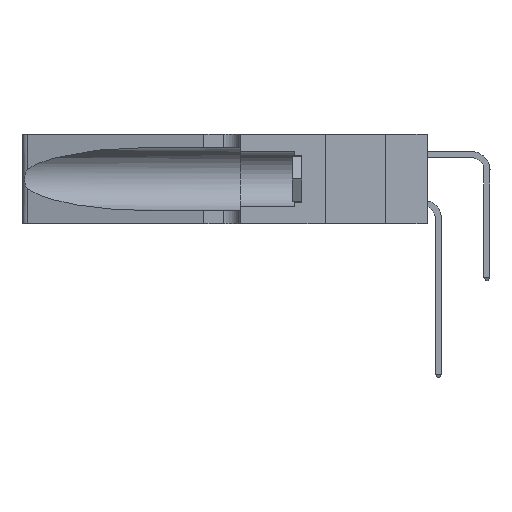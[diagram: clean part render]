
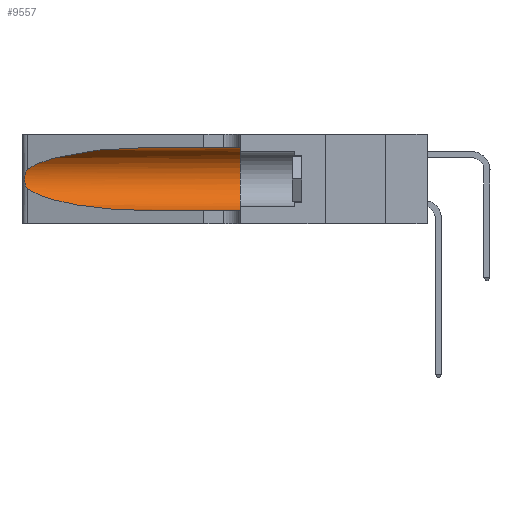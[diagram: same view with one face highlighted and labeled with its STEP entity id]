
A CAD part, left-side view. The second image highlights one B-rep face of the part: STEP entity #9557.
In plain terms, the highlighted cylindrical face has radius 3.308 mm (diameter 6.617 mm), a partial arc.
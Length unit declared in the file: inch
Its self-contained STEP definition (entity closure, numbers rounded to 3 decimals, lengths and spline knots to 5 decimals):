
#128 = DIRECTION ( 'NONE',  ( 0., -1., 0. ) ) ;
#168 = VERTEX_POINT ( 'NONE', #22204 ) ;
#1354 = CYLINDRICAL_SURFACE ( 'NONE', #5959, 0.13025 ) ;
#1761 = DIRECTION ( 'NONE',  ( 0., 1., 0. ) ) ;
#2140 = ORIENTED_EDGE ( 'NONE', *, *, #6679, .T. ) ;
#2148 = VERTEX_POINT ( 'NONE', #20950 ) ;
#2227 = CARTESIAN_POINT ( 'NONE',  ( 0.26018, 1.23835, 0.19895 ) ) ;
#3021 = VECTOR ( 'NONE', #128, 39.37008 ) ;
#3131 = DIRECTION ( 'NONE',  ( 0., 0., -1. ) ) ;
#3264 = VERTEX_POINT ( 'NONE', #19180 ) ;
#4527 = CARTESIAN_POINT ( 'NONE',  ( 0.25487, 1.22718, 0.22369 ) ) ;
#4631 = FACE_OUTER_BOUND ( 'NONE', #27424, .T. ) ;
#5343 =( BOUNDED_CURVE ( )  B_SPLINE_CURVE ( 3, ( #19104, #28848, #7785, #18140 ),
 .UNSPECIFIED., .F., .T. ) 
 B_SPLINE_CURVE_WITH_KNOTS ( ( 4, 4 ),
 ( 3.44316, 4.71239 ),
 .UNSPECIFIED. ) 
 CURVE ( )  GEOMETRIC_REPRESENTATION_ITEM ( )  RATIONAL_B_SPLINE_CURVE ( ( 1., 0.87, 0.87, 1. ) ) 
 REPRESENTATION_ITEM ( '' )  );
#5732 = CARTESIAN_POINT ( 'NONE',  ( 0.1305, 0.72297, 0.05475 ) ) ;
#5959 = AXIS2_PLACEMENT_3D ( 'NONE', #11702, #17139, #3131 ) ;
#6679 = EDGE_CURVE ( 'NONE', #9902, #25562, #5343, .T. ) ;
#6950 = CARTESIAN_POINT ( 'NONE',  ( 0.2373, 1.15595, 0.28018 ) ) ;
#7373 = CARTESIAN_POINT ( 'NONE',  ( 0.25856, 1.23593, 0.16098 ) ) ;
#7451 = CARTESIAN_POINT ( 'NONE',  ( 0.1305, 1.61858, 0.05475 ) ) ;
#7481 = ORIENTED_EDGE ( 'NONE', *, *, #14138, .T. ) ;
#7785 = CARTESIAN_POINT ( 'NONE',  ( 0.18966, 0.96281, 0.05475 ) ) ;
#9509 = CARTESIAN_POINT ( 'NONE',  ( 0.25639, 1.23184, 0.21858 ) ) ;
#9557 = ADVANCED_FACE ( 'NONE', ( #4631 ), #1354, .F. ) ;
#9620 = CARTESIAN_POINT ( 'NONE',  ( 0.25639, 1.23186, 0.15144 ) ) ;
#9720 = CARTESIAN_POINT ( 'NONE',  ( 0.25487, 1.22718, 0.22369 ) ) ;
#9807 = DIRECTION ( 'NONE',  ( 0., -1., 0. ) ) ;
#9902 = VERTEX_POINT ( 'NONE', #14813 ) ;
#10667 = ORIENTED_EDGE ( 'NONE', *, *, #11576, .T. ) ;
#10798 = CARTESIAN_POINT ( 'NONE',  ( 0.1305, 0.72297, 0.31525 ) ) ;
#10821 = EDGE_CURVE ( 'NONE', #3264, #2148, #24420, .T. ) ;
#11141 = CARTESIAN_POINT ( 'NONE',  ( 0.1305, 0.35, 0.185 ) ) ;
#11512 = ORIENTED_EDGE ( 'NONE', *, *, #13351, .T. ) ;
#11576 = EDGE_CURVE ( 'NONE', #19653, #9902, #26293, .T. ) ;
#11702 = CARTESIAN_POINT ( 'NONE',  ( 0.1305, 1.61858, 0.185 ) ) ;
#11894 = CARTESIAN_POINT ( 'NONE',  ( 0.26075, 1.23896, 0.19203 ) ) ;
#12830 = LINE ( 'NONE', #7451, #15030 ) ;
#13351 = EDGE_CURVE ( 'NONE', #168, #19653, #27240, .T. ) ;
#14138 = EDGE_CURVE ( 'NONE', #25562, #2148, #12830, .T. ) ;
#14353 = CARTESIAN_POINT ( 'NONE',  ( 0.26075, 1.23896, 0.178 ) ) ;
#14813 = CARTESIAN_POINT ( 'NONE',  ( 0.25487, 1.22718, 0.14631 ) ) ;
#15030 = VECTOR ( 'NONE', #9807, 39.37008 ) ;
#16624 = CARTESIAN_POINT ( 'NONE',  ( 0.25487, 1.22718, 0.14631 ) ) ;
#16697 = CARTESIAN_POINT ( 'NONE',  ( 0.18966, 0.96281, 0.31525 ) ) ;
#17139 = DIRECTION ( 'NONE',  ( 0., -1., 0. ) ) ;
#18140 = CARTESIAN_POINT ( 'NONE',  ( 0.1305, 0.72297, 0.05475 ) ) ;
#18201 = DIRECTION ( 'NONE',  ( 0., 0., 1. ) ) ;
#19048 = CARTESIAN_POINT ( 'NONE',  ( 0.1305, 1.61858, 0.31525 ) ) ;
#19104 = CARTESIAN_POINT ( 'NONE',  ( 0.25487, 1.22718, 0.14631 ) ) ;
#19180 = CARTESIAN_POINT ( 'NONE',  ( 0.1305, 0.35, 0.31525 ) ) ;
#19653 = VERTEX_POINT ( 'NONE', #4527 ) ;
#20950 = CARTESIAN_POINT ( 'NONE',  ( 0.1305, 0.35, 0.05475 ) ) ;
#21390 = CARTESIAN_POINT ( 'NONE',  ( 0.25555, 1.22993, 0.14849 ) ) ;
#21469 = CARTESIAN_POINT ( 'NONE',  ( 0.26017, 1.23833, 0.17102 ) ) ;
#22050 = ORIENTED_EDGE ( 'NONE', *, *, #27349, .F. ) ;
#22204 = CARTESIAN_POINT ( 'NONE',  ( 0.1305, 0.72297, 0.31525 ) ) ;
#22681 = ORIENTED_EDGE ( 'NONE', *, *, #10821, .F. ) ;
#23428 = CARTESIAN_POINT ( 'NONE',  ( 0.25787, 1.23484, 0.2124 ) ) ;
#24420 = CIRCLE ( 'NONE', #25694, 0.13025 ) ;
#25424 = CARTESIAN_POINT ( 'NONE',  ( 0.25487, 1.22718, 0.22369 ) ) ;
#25562 = VERTEX_POINT ( 'NONE', #5732 ) ;
#25694 = AXIS2_PLACEMENT_3D ( 'NONE', #11141, #1761, #18201 ) ;
#26076 = CARTESIAN_POINT ( 'NONE',  ( 0.25555, 1.22994, 0.2215 ) ) ;
#26293 = B_SPLINE_CURVE_WITH_KNOTS ( 'NONE', 3,
 ( #9720, #26076, #9509, #23428, #28422, #2227, #11894, #14353, #21469, #7373, #28130, #9620, #21390, #16624 ),
 .UNSPECIFIED., .F., .F.,
 ( 4, 2, 2, 2, 2, 2, 4 ),
 ( 0., 0.00027, 0.00053, 0.00107, 0.0016, 0.00187, 0.00214 ),
 .UNSPECIFIED. ) ;
#27240 =( BOUNDED_CURVE ( )  B_SPLINE_CURVE ( 3, ( #10798, #16697, #6950, #25424 ),
 .UNSPECIFIED., .F., .T. ) 
 B_SPLINE_CURVE_WITH_KNOTS ( ( 4, 4 ),
 ( 1.5708, 2.84003 ),
 .UNSPECIFIED. ) 
 CURVE ( )  GEOMETRIC_REPRESENTATION_ITEM ( )  RATIONAL_B_SPLINE_CURVE ( ( 1., 0.87, 0.87, 1. ) ) 
 REPRESENTATION_ITEM ( '' )  );
#27315 = LINE ( 'NONE', #19048, #3021 ) ;
#27349 = EDGE_CURVE ( 'NONE', #168, #3264, #27315, .T. ) ;
#27424 = EDGE_LOOP ( 'NONE', ( #11512, #10667, #2140, #7481, #22681, #22050 ) ) ;
#28130 = CARTESIAN_POINT ( 'NONE',  ( 0.25789, 1.23486, 0.15765 ) ) ;
#28422 = CARTESIAN_POINT ( 'NONE',  ( 0.25854, 1.2359, 0.20912 ) ) ;
#28848 = CARTESIAN_POINT ( 'NONE',  ( 0.2373, 1.15595, 0.08982 ) ) ;
